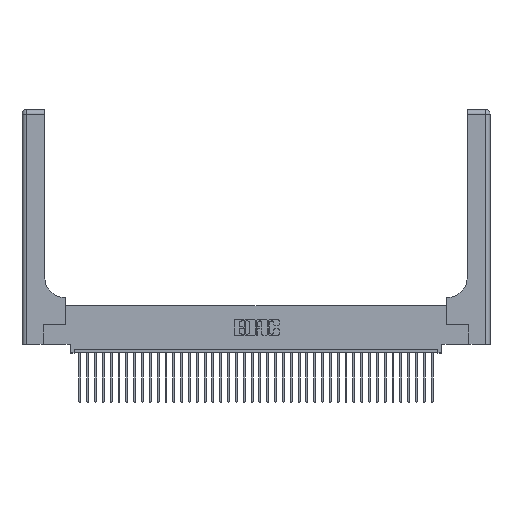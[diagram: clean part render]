
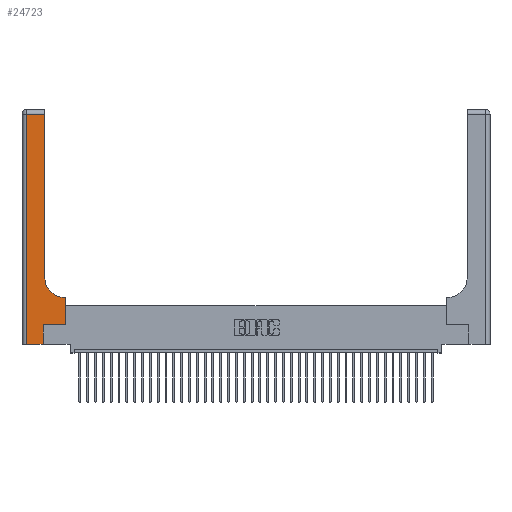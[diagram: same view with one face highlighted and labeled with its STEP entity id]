
A CAD part, top view. The second image highlights one B-rep face of the part: STEP entity #24723.
In plain terms, the highlighted planar face has unit normal (0, 0, 1).
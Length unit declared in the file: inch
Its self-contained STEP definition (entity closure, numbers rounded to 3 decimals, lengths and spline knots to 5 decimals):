
#1214 = DIRECTION ( 'NONE',  ( -1., 0., 0. ) ) ;
#1902 = CARTESIAN_POINT ( 'NONE',  ( 0.5415, 0.85, 0.37 ) ) ;
#1928 = CARTESIAN_POINT ( 'NONE',  ( 0., 3., 0.37 ) ) ;
#2058 = DIRECTION ( 'NONE',  ( -1., 0., 0. ) ) ;
#2146 = LINE ( 'NONE', #32532, #32649 ) ;
#2581 = CIRCLE ( 'NONE', #10649, 0.25 ) ;
#2698 = VERTEX_POINT ( 'NONE', #19209 ) ;
#3000 = LINE ( 'NONE', #10873, #3444 ) ;
#3444 = VECTOR ( 'NONE', #19940, 39.37008 ) ;
#3668 = LINE ( 'NONE', #14077, #6562 ) ;
#3925 = VERTEX_POINT ( 'NONE', #16904 ) ;
#4045 = LINE ( 'NONE', #28102, #33594 ) ;
#5660 = CARTESIAN_POINT ( 'NONE',  ( 0.269, 0., 0.37 ) ) ;
#6118 = VERTEX_POINT ( 'NONE', #9114 ) ;
#6562 = VECTOR ( 'NONE', #10890, 39.37008 ) ;
#7626 = CARTESIAN_POINT ( 'NONE',  ( 0.2915, 0.6, 0.37 ) ) ;
#8706 = CARTESIAN_POINT ( 'NONE',  ( 0.06, 2.94, 0.37 ) ) ;
#9114 = CARTESIAN_POINT ( 'NONE',  ( 0.2915, 0.85, 0.37 ) ) ;
#9554 = VECTOR ( 'NONE', #11651, 39.37008 ) ;
#9876 = CARTESIAN_POINT ( 'NONE',  ( 0.2915, 2.94, 0.37 ) ) ;
#10202 = DIRECTION ( 'NONE',  ( -1., 0., 0. ) ) ;
#10579 = EDGE_CURVE ( 'NONE', #21477, #29215, #2146, .T. ) ;
#10612 = LINE ( 'NONE', #7626, #34925 ) ;
#10649 = AXIS2_PLACEMENT_3D ( 'NONE', #1902, #20025, #14014 ) ;
#10873 = CARTESIAN_POINT ( 'NONE',  ( 0.06, 3., 0.37 ) ) ;
#10890 = DIRECTION ( 'NONE',  ( 0., 1., 0. ) ) ;
#11651 = DIRECTION ( 'NONE',  ( 0., 1., 0. ) ) ;
#13623 = CARTESIAN_POINT ( 'NONE',  ( 0.5585, 0.6, 0.37 ) ) ;
#14014 = DIRECTION ( 'NONE',  ( 1., 0., 0. ) ) ;
#14077 = CARTESIAN_POINT ( 'NONE',  ( 0.5585, 0.25, 0.37 ) ) ;
#14366 = EDGE_CURVE ( 'NONE', #25628, #37664, #10612, .T. ) ;
#15104 = ORIENTED_EDGE ( 'NONE', *, *, #36734, .T. ) ;
#15267 = LINE ( 'NONE', #5660, #31982 ) ;
#15380 = ORIENTED_EDGE ( 'NONE', *, *, #34159, .T. ) ;
#16770 = VERTEX_POINT ( 'NONE', #9876 ) ;
#16904 = CARTESIAN_POINT ( 'NONE',  ( 0.06, 0., 0.37 ) ) ;
#18508 = LINE ( 'NONE', #36410, #27999 ) ;
#18892 = ORIENTED_EDGE ( 'NONE', *, *, #10579, .T. ) ;
#19209 = CARTESIAN_POINT ( 'NONE',  ( 0.269, 0., 0.37 ) ) ;
#19815 = FACE_OUTER_BOUND ( 'NONE', #34800, .T. ) ;
#19940 = DIRECTION ( 'NONE',  ( 0., -1., 0. ) ) ;
#20025 = DIRECTION ( 'NONE',  ( 0., 0., -1. ) ) ;
#20154 = ORIENTED_EDGE ( 'NONE', *, *, #20200, .T. ) ;
#20200 = EDGE_CURVE ( 'NONE', #37664, #6118, #2581, .T. ) ;
#21477 = VERTEX_POINT ( 'NONE', #39294 ) ;
#21613 = CARTESIAN_POINT ( 'NONE',  ( 0.5585, 0.25, 0.37 ) ) ;
#21720 = DIRECTION ( 'NONE',  ( 1., 0., 0. ) ) ;
#21824 = ORIENTED_EDGE ( 'NONE', *, *, #21977, .T. ) ;
#21977 = EDGE_CURVE ( 'NONE', #2698, #21477, #15267, .T. ) ;
#22929 = EDGE_CURVE ( 'NONE', #16770, #23977, #18508, .T. ) ;
#23297 = EDGE_CURVE ( 'NONE', #29215, #25628, #3668, .T. ) ;
#23977 = VERTEX_POINT ( 'NONE', #8706 ) ;
#24723 = ADVANCED_FACE ( 'NONE', ( #19815 ), #38368, .F. ) ;
#25044 = ORIENTED_EDGE ( 'NONE', *, *, #38114, .T. ) ;
#25628 = VERTEX_POINT ( 'NONE', #13623 ) ;
#27818 = ORIENTED_EDGE ( 'NONE', *, *, #22929, .T. ) ;
#27999 = VECTOR ( 'NONE', #10202, 39.37008 ) ;
#28078 = ORIENTED_EDGE ( 'NONE', *, *, #23297, .T. ) ;
#28102 = CARTESIAN_POINT ( 'NONE',  ( 0., 0., 0.37 ) ) ;
#28365 = DIRECTION ( 'NONE',  ( 0., 1., 0. ) ) ;
#29215 = VERTEX_POINT ( 'NONE', #21613 ) ;
#29906 = CARTESIAN_POINT ( 'NONE',  ( 0.2915, 3., 0.37 ) ) ;
#31982 = VECTOR ( 'NONE', #28365, 39.37008 ) ;
#32532 = CARTESIAN_POINT ( 'NONE',  ( 0.269, 0.25, 0.37 ) ) ;
#32649 = VECTOR ( 'NONE', #34323, 39.37008 ) ;
#32708 = AXIS2_PLACEMENT_3D ( 'NONE', #1928, #35727, #2058 ) ;
#33289 = CARTESIAN_POINT ( 'NONE',  ( 0.5415, 0.6, 0.37 ) ) ;
#33419 = LINE ( 'NONE', #29906, #9554 ) ;
#33594 = VECTOR ( 'NONE', #21720, 39.37008 ) ;
#34159 = EDGE_CURVE ( 'NONE', #6118, #16770, #33419, .T. ) ;
#34323 = DIRECTION ( 'NONE',  ( 1., 0., 0. ) ) ;
#34800 = EDGE_LOOP ( 'NONE', ( #15380, #27818, #25044, #15104, #21824, #18892, #28078, #37443, #20154 ) ) ;
#34925 = VECTOR ( 'NONE', #1214, 39.37008 ) ;
#35727 = DIRECTION ( 'NONE',  ( 0., 0., -1. ) ) ;
#36410 = CARTESIAN_POINT ( 'NONE',  ( 0., 2.94, 0.37 ) ) ;
#36734 = EDGE_CURVE ( 'NONE', #3925, #2698, #4045, .T. ) ;
#37443 = ORIENTED_EDGE ( 'NONE', *, *, #14366, .T. ) ;
#37664 = VERTEX_POINT ( 'NONE', #33289 ) ;
#38114 = EDGE_CURVE ( 'NONE', #23977, #3925, #3000, .T. ) ;
#38368 = PLANE ( 'NONE',  #32708 ) ;
#39294 = CARTESIAN_POINT ( 'NONE',  ( 0.269, 0.25, 0.37 ) ) ;
